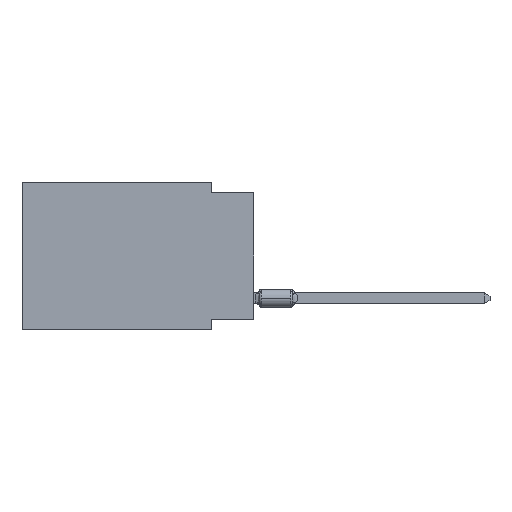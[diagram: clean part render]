
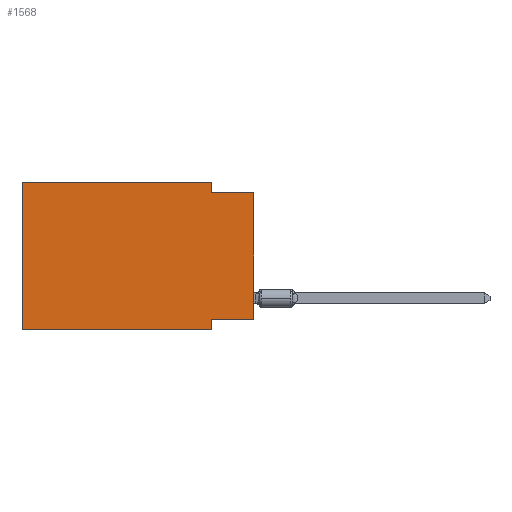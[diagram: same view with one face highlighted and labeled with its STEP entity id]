
A CAD part, left-side view. The second image highlights one B-rep face of the part: STEP entity #1568.
In plain terms, the highlighted planar face has unit normal (-1, 0, 0).
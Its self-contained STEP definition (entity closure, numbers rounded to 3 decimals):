
#33 = CARTESIAN_POINT ( 'NONE',  ( 0., 13.97, 0. ) ) ;
#147 = DIRECTION ( 'NONE',  ( 0., 0., -1. ) ) ;
#835 = DIRECTION ( 'NONE',  ( 0., 0., 1. ) ) ;
#848 = VERTEX_POINT ( 'NONE', #14474 ) ;
#924 = EDGE_CURVE ( 'NONE', #11479, #17952, #10026, .T. ) ;
#1223 = CARTESIAN_POINT ( 'NONE',  ( 0., 13.97, -8.89 ) ) ;
#1568 = ADVANCED_FACE ( 'NONE', ( #2747 ), #2192, .F. ) ;
#2050 = EDGE_CURVE ( 'NONE', #6717, #22984, #21071, .T. ) ;
#2192 = PLANE ( 'NONE',  #26288 ) ;
#2321 = DIRECTION ( 'NONE',  ( 0., 0., -1. ) ) ;
#2470 = DIRECTION ( 'NONE',  ( 0., -1., 0. ) ) ;
#2679 = ORIENTED_EDGE ( 'NONE', *, *, #924, .T. ) ;
#2747 = FACE_OUTER_BOUND ( 'NONE', #25314, .T. ) ;
#3029 = ORIENTED_EDGE ( 'NONE', *, *, #7520, .F. ) ;
#3691 = CARTESIAN_POINT ( 'NONE',  ( 0., 2.54, -8.89 ) ) ;
#5110 = VECTOR ( 'NONE', #13565, 1000. ) ;
#5175 = VERTEX_POINT ( 'NONE', #22647 ) ;
#6717 = VERTEX_POINT ( 'NONE', #27493 ) ;
#6971 = DIRECTION ( 'NONE',  ( 0., -1., 0. ) ) ;
#7520 = EDGE_CURVE ( 'NONE', #24993, #22984, #27565, .T. ) ;
#7579 = CARTESIAN_POINT ( 'NONE',  ( 0., 0., -8.255 ) ) ;
#7866 = LINE ( 'NONE', #7579, #24400 ) ;
#8819 = DIRECTION ( 'NONE',  ( 1., 0., 0. ) ) ;
#8883 = ORIENTED_EDGE ( 'NONE', *, *, #19221, .F. ) ;
#9880 = CARTESIAN_POINT ( 'NONE',  ( 0., 0., 0. ) ) ;
#10026 = LINE ( 'NONE', #9880, #10926 ) ;
#10393 = CARTESIAN_POINT ( 'NONE',  ( 0., 2.54, -8.255 ) ) ;
#10641 = CARTESIAN_POINT ( 'NONE',  ( 0., 0., -0.635 ) ) ;
#10794 = LINE ( 'NONE', #15389, #15910 ) ;
#10926 = VECTOR ( 'NONE', #835, 1000. ) ;
#10975 = CARTESIAN_POINT ( 'NONE',  ( 0., 0., -0.635 ) ) ;
#10992 = VECTOR ( 'NONE', #11875, 1000. ) ;
#11214 = ORIENTED_EDGE ( 'NONE', *, *, #23423, .F. ) ;
#11479 = VERTEX_POINT ( 'NONE', #25550 ) ;
#11875 = DIRECTION ( 'NONE',  ( 0., -1., 0. ) ) ;
#12170 = DIRECTION ( 'NONE',  ( 0., 1., 0. ) ) ;
#12449 = DIRECTION ( 'NONE',  ( 0., 0., -1. ) ) ;
#13565 = DIRECTION ( 'NONE',  ( 0., 0., 1. ) ) ;
#14176 = EDGE_CURVE ( 'NONE', #11479, #24993, #7866, .T. ) ;
#14440 = VECTOR ( 'NONE', #2470, 1000. ) ;
#14474 = CARTESIAN_POINT ( 'NONE',  ( 0., 2.54, -0.635 ) ) ;
#14827 = EDGE_CURVE ( 'NONE', #6717, #21766, #26801, .T. ) ;
#15389 = CARTESIAN_POINT ( 'NONE',  ( 0., 2.54, 0. ) ) ;
#15609 = CARTESIAN_POINT ( 'NONE',  ( 0., 13.97, 0. ) ) ;
#15877 = CARTESIAN_POINT ( 'NONE',  ( 0., 2.54, -8.89 ) ) ;
#15910 = VECTOR ( 'NONE', #147, 1000. ) ;
#16430 = VECTOR ( 'NONE', #6971, 1000. ) ;
#16601 = ORIENTED_EDGE ( 'NONE', *, *, #2050, .T. ) ;
#17952 = VERTEX_POINT ( 'NONE', #10641 ) ;
#19221 = EDGE_CURVE ( 'NONE', #5175, #848, #10794, .T. ) ;
#21071 = LINE ( 'NONE', #1223, #10992 ) ;
#21639 = CARTESIAN_POINT ( 'NONE',  ( 0., 13.97, 0. ) ) ;
#21766 = VERTEX_POINT ( 'NONE', #21639 ) ;
#22178 = LINE ( 'NONE', #10975, #14440 ) ;
#22647 = CARTESIAN_POINT ( 'NONE',  ( 0., 2.54, 0. ) ) ;
#22984 = VERTEX_POINT ( 'NONE', #15877 ) ;
#23159 = ORIENTED_EDGE ( 'NONE', *, *, #14176, .F. ) ;
#23423 = EDGE_CURVE ( 'NONE', #848, #17952, #22178, .T. ) ;
#24190 = VECTOR ( 'NONE', #12449, 1000. ) ;
#24226 = CARTESIAN_POINT ( 'NONE',  ( 0., 13.97, 0. ) ) ;
#24400 = VECTOR ( 'NONE', #12170, 1000. ) ;
#24993 = VERTEX_POINT ( 'NONE', #10393 ) ;
#25314 = EDGE_LOOP ( 'NONE', ( #2679, #11214, #8883, #27235, #25687, #16601, #3029, #23159 ) ) ;
#25550 = CARTESIAN_POINT ( 'NONE',  ( 0., 0., -8.255 ) ) ;
#25687 = ORIENTED_EDGE ( 'NONE', *, *, #14827, .F. ) ;
#25904 = EDGE_CURVE ( 'NONE', #21766, #5175, #28425, .T. ) ;
#26288 = AXIS2_PLACEMENT_3D ( 'NONE', #33, #8819, #2321 ) ;
#26801 = LINE ( 'NONE', #24226, #5110 ) ;
#27235 = ORIENTED_EDGE ( 'NONE', *, *, #25904, .F. ) ;
#27493 = CARTESIAN_POINT ( 'NONE',  ( 0., 13.97, -8.89 ) ) ;
#27565 = LINE ( 'NONE', #3691, #24190 ) ;
#28425 = LINE ( 'NONE', #15609, #16430 ) ;
